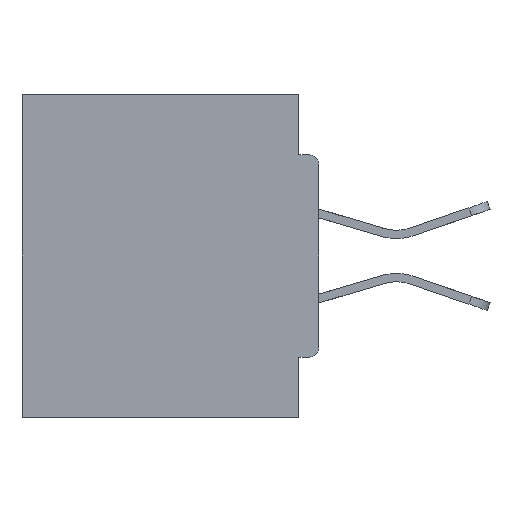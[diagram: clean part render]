
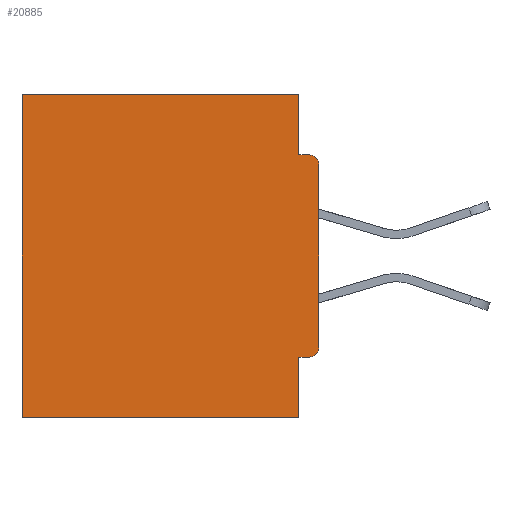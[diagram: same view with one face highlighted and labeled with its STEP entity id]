
A CAD part, left-side view. The second image highlights one B-rep face of the part: STEP entity #20885.
In plain terms, the highlighted planar face has unit normal (-1, 0, 0).
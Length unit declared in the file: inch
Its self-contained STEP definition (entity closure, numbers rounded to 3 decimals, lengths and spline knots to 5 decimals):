
#78 = ORIENTED_EDGE ( 'NONE', *, *, #8814, .T. ) ;
#238 = EDGE_CURVE ( 'NONE', #23391, #31837, #31452, .T. ) ;
#775 = CARTESIAN_POINT ( 'NONE',  ( 0.298, 0.015, -0.4065 ) ) ;
#1490 = VECTOR ( 'NONE', #25771, 39.37008 ) ;
#2139 = ORIENTED_EDGE ( 'NONE', *, *, #2319, .T. ) ;
#2274 = CARTESIAN_POINT ( 'NONE',  ( 0.298, 0., 0. ) ) ;
#2319 = EDGE_CURVE ( 'NONE', #26339, #32025, #32977, .T. ) ;
#2588 = DIRECTION ( 'NONE',  ( 0., -1., 0. ) ) ;
#2971 = CARTESIAN_POINT ( 'NONE',  ( 0.298, 0., -0.1085 ) ) ;
#2978 = CARTESIAN_POINT ( 'NONE',  ( 0.298, 0., 0. ) ) ;
#3910 = EDGE_CURVE ( 'NONE', #11598, #27125, #21677, .T. ) ;
#4421 = VECTOR ( 'NONE', #31683, 39.37008 ) ;
#5147 = EDGE_CURVE ( 'NONE', #10448, #31907, #25411, .T. ) ;
#5502 = ORIENTED_EDGE ( 'NONE', *, *, #21487, .F. ) ;
#7684 = EDGE_CURVE ( 'NONE', #23391, #27968, #26894, .T. ) ;
#7694 = VERTEX_POINT ( 'NONE', #13414 ) ;
#8653 = DIRECTION ( 'NONE',  ( 0., 0., -1. ) ) ;
#8814 = EDGE_CURVE ( 'NONE', #31837, #7694, #17235, .T. ) ;
#9028 = DIRECTION ( 'NONE',  ( 0., 0., -1. ) ) ;
#9234 = CARTESIAN_POINT ( 'NONE',  ( 0.298, 0., -0.3915 ) ) ;
#9614 = CARTESIAN_POINT ( 'NONE',  ( 0.298, 0.031, -0.5 ) ) ;
#9874 = LINE ( 'NONE', #15766, #30578 ) ;
#9900 = CARTESIAN_POINT ( 'NONE',  ( 0.298, 0., -0.4065 ) ) ;
#10062 = CARTESIAN_POINT ( 'NONE',  ( 0.298, 0.46, 0. ) ) ;
#10063 = VECTOR ( 'NONE', #33948, 39.37008 ) ;
#10128 = PLANE ( 'NONE',  #10518 ) ;
#10448 = VERTEX_POINT ( 'NONE', #29728 ) ;
#10518 = AXIS2_PLACEMENT_3D ( 'NONE', #2274, #23445, #15122 ) ;
#11598 = VERTEX_POINT ( 'NONE', #2971 ) ;
#11816 = CARTESIAN_POINT ( 'NONE',  ( 0.298, 0.031, -0.5 ) ) ;
#11926 = ORIENTED_EDGE ( 'NONE', *, *, #32994, .F. ) ;
#13414 = CARTESIAN_POINT ( 'NONE',  ( 0.298, 0.46, -0.5 ) ) ;
#14647 = ORIENTED_EDGE ( 'NONE', *, *, #30148, .F. ) ;
#15070 = ORIENTED_EDGE ( 'NONE', *, *, #7684, .F. ) ;
#15122 = DIRECTION ( 'NONE',  ( 0., 0., -1. ) ) ;
#15442 = LINE ( 'NONE', #34303, #10063 ) ;
#15766 = CARTESIAN_POINT ( 'NONE',  ( 0.298, 0., -0.0935 ) ) ;
#17235 = LINE ( 'NONE', #10062, #4421 ) ;
#18011 = ORIENTED_EDGE ( 'NONE', *, *, #19776, .F. ) ;
#18187 = CARTESIAN_POINT ( 'NONE',  ( 0.298, 0.031, 0. ) ) ;
#18934 = CARTESIAN_POINT ( 'NONE',  ( 0.298, 0.031, -0.0935 ) ) ;
#19223 = CARTESIAN_POINT ( 'NONE',  ( 0.298, 0.015, -0.3915 ) ) ;
#19575 = LINE ( 'NONE', #25376, #26591 ) ;
#19776 = EDGE_CURVE ( 'NONE', #26339, #10448, #30865, .T. ) ;
#20682 = VECTOR ( 'NONE', #8653, 39.37008 ) ;
#20885 = ADVANCED_FACE ( 'NONE', ( #33696 ), #10128, .F. ) ;
#20893 = VECTOR ( 'NONE', #9028, 39.37008 ) ;
#21487 = EDGE_CURVE ( 'NONE', #11598, #32025, #15442, .T. ) ;
#21540 = VECTOR ( 'NONE', #32118, 39.37008 ) ;
#21677 = CIRCLE ( 'NONE', #23648, 0.015 ) ;
#21698 = ORIENTED_EDGE ( 'NONE', *, *, #238, .T. ) ;
#21768 = CARTESIAN_POINT ( 'NONE',  ( 0.298, 0.015, -0.1085 ) ) ;
#23391 = VERTEX_POINT ( 'NONE', #18187 ) ;
#23442 = CARTESIAN_POINT ( 'NONE',  ( 0.298, 0.015, -0.0935 ) ) ;
#23445 = DIRECTION ( 'NONE',  ( 1., 0., 0. ) ) ;
#23648 = AXIS2_PLACEMENT_3D ( 'NONE', #21768, #24778, #27209 ) ;
#24512 = CARTESIAN_POINT ( 'NONE',  ( 0.298, 0.031, -0.5 ) ) ;
#24543 = DIRECTION ( 'NONE',  ( -1., 0., 0. ) ) ;
#24778 = DIRECTION ( 'NONE',  ( -1., 0., 0. ) ) ;
#25376 = CARTESIAN_POINT ( 'NONE',  ( 0.298, 0., -0.5 ) ) ;
#25411 = LINE ( 'NONE', #11816, #20893 ) ;
#25771 = DIRECTION ( 'NONE',  ( 0., 1., 0. ) ) ;
#26339 = VERTEX_POINT ( 'NONE', #775 ) ;
#26591 = VECTOR ( 'NONE', #28029, 39.37008 ) ;
#26894 = LINE ( 'NONE', #24512, #20682 ) ;
#27125 = VERTEX_POINT ( 'NONE', #23442 ) ;
#27209 = DIRECTION ( 'NONE',  ( 0., 0., -1. ) ) ;
#27314 = DIRECTION ( 'NONE',  ( 0., 0., -1. ) ) ;
#27968 = VERTEX_POINT ( 'NONE', #18934 ) ;
#28028 = ORIENTED_EDGE ( 'NONE', *, *, #3910, .T. ) ;
#28029 = DIRECTION ( 'NONE',  ( 0., 1., 0. ) ) ;
#28241 = CARTESIAN_POINT ( 'NONE',  ( 0.298, 0.46, 0. ) ) ;
#29163 = AXIS2_PLACEMENT_3D ( 'NONE', #19223, #24543, #27314 ) ;
#29728 = CARTESIAN_POINT ( 'NONE',  ( 0.298, 0.031, -0.4065 ) ) ;
#30148 = EDGE_CURVE ( 'NONE', #31907, #7694, #19575, .T. ) ;
#30260 = EDGE_LOOP ( 'NONE', ( #28028, #11926, #15070, #21698, #78, #14647, #30741, #18011, #2139, #5502 ) ) ;
#30578 = VECTOR ( 'NONE', #2588, 39.37008 ) ;
#30741 = ORIENTED_EDGE ( 'NONE', *, *, #5147, .F. ) ;
#30865 = LINE ( 'NONE', #9900, #1490 ) ;
#31452 = LINE ( 'NONE', #2978, #21540 ) ;
#31683 = DIRECTION ( 'NONE',  ( 0., 0., -1. ) ) ;
#31837 = VERTEX_POINT ( 'NONE', #28241 ) ;
#31907 = VERTEX_POINT ( 'NONE', #9614 ) ;
#32025 = VERTEX_POINT ( 'NONE', #9234 ) ;
#32118 = DIRECTION ( 'NONE',  ( 0., 1., 0. ) ) ;
#32977 = CIRCLE ( 'NONE', #29163, 0.015 ) ;
#32994 = EDGE_CURVE ( 'NONE', #27968, #27125, #9874, .T. ) ;
#33696 = FACE_OUTER_BOUND ( 'NONE', #30260, .T. ) ;
#33948 = DIRECTION ( 'NONE',  ( 0., 0., -1. ) ) ;
#34303 = CARTESIAN_POINT ( 'NONE',  ( 0.298, 0., 0. ) ) ;
